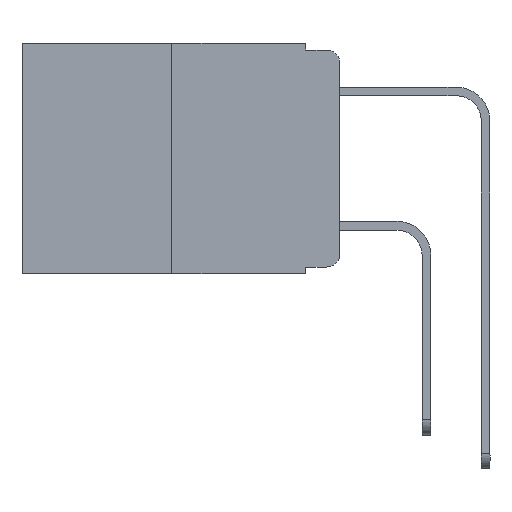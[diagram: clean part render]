
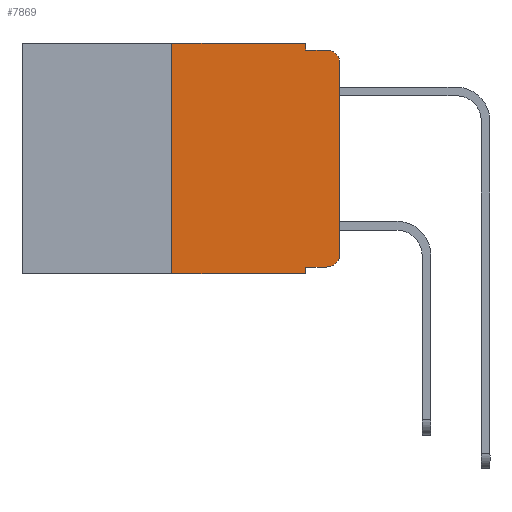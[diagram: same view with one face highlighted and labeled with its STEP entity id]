
A CAD part, left-side view. The second image highlights one B-rep face of the part: STEP entity #7869.
In plain terms, the highlighted planar face has unit normal (-1, 0, 0).
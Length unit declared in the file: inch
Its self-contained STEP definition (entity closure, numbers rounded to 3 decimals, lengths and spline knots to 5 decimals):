
#255 = VERTEX_POINT ( 'NONE', #11328 ) ;
#320 = CARTESIAN_POINT ( 'NONE',  ( 0., 0., -0.03 ) ) ;
#586 = LINE ( 'NONE', #3734, #12465 ) ;
#1014 = CARTESIAN_POINT ( 'NONE',  ( 0., 0.473, 0. ) ) ;
#1175 = VERTEX_POINT ( 'NONE', #11991 ) ;
#1264 = DIRECTION ( 'NONE',  ( 0., 0., -1. ) ) ;
#1426 = CARTESIAN_POINT ( 'NONE',  ( 0., 0.051, 0. ) ) ;
#1938 = VERTEX_POINT ( 'NONE', #16178 ) ;
#1976 = VERTEX_POINT ( 'NONE', #9786 ) ;
#2070 = ORIENTED_EDGE ( 'NONE', *, *, #16264, .F. ) ;
#2520 = VERTEX_POINT ( 'NONE', #320 ) ;
#2596 = CARTESIAN_POINT ( 'NONE',  ( 0., 0.473, 0. ) ) ;
#2667 = CARTESIAN_POINT ( 'NONE',  ( 0., 0.051, -0.01 ) ) ;
#2945 = DIRECTION ( 'NONE',  ( 0., -1., 0. ) ) ;
#3624 = VERTEX_POINT ( 'NONE', #10692 ) ;
#3734 = CARTESIAN_POINT ( 'NONE',  ( 0., 0.473, -0.343 ) ) ;
#3740 = DIRECTION ( 'NONE',  ( 0., 0., 1. ) ) ;
#4158 = VERTEX_POINT ( 'NONE', #15428 ) ;
#4434 = EDGE_CURVE ( 'NONE', #2520, #18762, #13626, .T. ) ;
#4568 = DIRECTION ( 'NONE',  ( 0., 0., -1. ) ) ;
#5041 = AXIS2_PLACEMENT_3D ( 'NONE', #15150, #12114, #19745 ) ;
#5365 = LINE ( 'NONE', #19301, #5650 ) ;
#5607 = DIRECTION ( 'NONE',  ( 0., -1., 0. ) ) ;
#5650 = VECTOR ( 'NONE', #7187, 39.37008 ) ;
#6432 = CARTESIAN_POINT ( 'NONE',  ( 0., 0.051, 0. ) ) ;
#6876 = EDGE_CURVE ( 'NONE', #10202, #1938, #14344, .T. ) ;
#7014 = EDGE_CURVE ( 'NONE', #1938, #18762, #8453, .T. ) ;
#7187 = DIRECTION ( 'NONE',  ( 0., 0., 1. ) ) ;
#7229 = ORIENTED_EDGE ( 'NONE', *, *, #7014, .F. ) ;
#7869 = ADVANCED_FACE ( 'NONE', ( #17148 ), #15623, .F. ) ;
#8090 = ORIENTED_EDGE ( 'NONE', *, *, #10468, .T. ) ;
#8453 = LINE ( 'NONE', #2667, #16938 ) ;
#9016 = VECTOR ( 'NONE', #3740, 39.37008 ) ;
#9132 = LINE ( 'NONE', #13785, #12609 ) ;
#9181 = DIRECTION ( 'NONE',  ( 0., -1., 0. ) ) ;
#9277 = ORIENTED_EDGE ( 'NONE', *, *, #6876, .F. ) ;
#9786 = CARTESIAN_POINT ( 'NONE',  ( 0., 0.25, 0. ) ) ;
#10202 = VERTEX_POINT ( 'NONE', #1426 ) ;
#10287 = CARTESIAN_POINT ( 'NONE',  ( 0., 0.02, -0.01 ) ) ;
#10468 = EDGE_CURVE ( 'NONE', #255, #4158, #586, .T. ) ;
#10527 = EDGE_CURVE ( 'NONE', #18423, #2520, #5365, .T. ) ;
#10692 = CARTESIAN_POINT ( 'NONE',  ( 0., 0.051, -0.333 ) ) ;
#10819 = CARTESIAN_POINT ( 'NONE',  ( 0., 0., -0.313 ) ) ;
#11205 = CIRCLE ( 'NONE', #5041, 0.02 ) ;
#11256 = ORIENTED_EDGE ( 'NONE', *, *, #19028, .F. ) ;
#11328 = CARTESIAN_POINT ( 'NONE',  ( 0., 0.25, -0.343 ) ) ;
#11362 = DIRECTION ( 'NONE',  ( -1., 0., 0. ) ) ;
#11364 = CARTESIAN_POINT ( 'NONE',  ( 0., 0.25, 0. ) ) ;
#11454 = CARTESIAN_POINT ( 'NONE',  ( 0., 0.02, -0.03 ) ) ;
#11749 = EDGE_CURVE ( 'NONE', #1175, #18423, #11205, .T. ) ;
#11991 = CARTESIAN_POINT ( 'NONE',  ( 0., 0.02, -0.333 ) ) ;
#12114 = DIRECTION ( 'NONE',  ( -1., 0., 0. ) ) ;
#12314 = ORIENTED_EDGE ( 'NONE', *, *, #17540, .F. ) ;
#12465 = VECTOR ( 'NONE', #12985, 39.37008 ) ;
#12473 = ORIENTED_EDGE ( 'NONE', *, *, #10527, .T. ) ;
#12609 = VECTOR ( 'NONE', #4568, 39.37008 ) ;
#12985 = DIRECTION ( 'NONE',  ( 0., -1., 0. ) ) ;
#13444 = LINE ( 'NONE', #19660, #14844 ) ;
#13626 = CIRCLE ( 'NONE', #13940, 0.02 ) ;
#13785 = CARTESIAN_POINT ( 'NONE',  ( 0., 0.051, 0. ) ) ;
#13940 = AXIS2_PLACEMENT_3D ( 'NONE', #11454, #11362, #16026 ) ;
#14017 = VECTOR ( 'NONE', #18837, 39.37008 ) ;
#14344 = LINE ( 'NONE', #6432, #14017 ) ;
#14844 = VECTOR ( 'NONE', #9181, 39.37008 ) ;
#15150 = CARTESIAN_POINT ( 'NONE',  ( 0., 0.02, -0.313 ) ) ;
#15269 = EDGE_CURVE ( 'NONE', #3624, #1175, #13444, .T. ) ;
#15335 = AXIS2_PLACEMENT_3D ( 'NONE', #2596, #18141, #1264 ) ;
#15428 = CARTESIAN_POINT ( 'NONE',  ( 0., 0.051, -0.343 ) ) ;
#15623 = PLANE ( 'NONE',  #15335 ) ;
#16026 = DIRECTION ( 'NONE',  ( 0., 0., -1. ) ) ;
#16100 = VECTOR ( 'NONE', #2945, 39.37008 ) ;
#16178 = CARTESIAN_POINT ( 'NONE',  ( 0., 0.051, -0.01 ) ) ;
#16264 = EDGE_CURVE ( 'NONE', #3624, #4158, #9132, .T. ) ;
#16657 = LINE ( 'NONE', #1014, #16100 ) ;
#16938 = VECTOR ( 'NONE', #5607, 39.37008 ) ;
#17087 = ORIENTED_EDGE ( 'NONE', *, *, #11749, .T. ) ;
#17148 = FACE_OUTER_BOUND ( 'NONE', #19025, .T. ) ;
#17540 = EDGE_CURVE ( 'NONE', #1976, #10202, #16657, .T. ) ;
#17725 = ORIENTED_EDGE ( 'NONE', *, *, #4434, .T. ) ;
#18141 = DIRECTION ( 'NONE',  ( 1., 0., 0. ) ) ;
#18423 = VERTEX_POINT ( 'NONE', #10819 ) ;
#18762 = VERTEX_POINT ( 'NONE', #10287 ) ;
#18837 = DIRECTION ( 'NONE',  ( 0., 0., -1. ) ) ;
#19025 = EDGE_LOOP ( 'NONE', ( #12473, #17725, #7229, #9277, #12314, #11256, #8090, #2070, #19159, #17087 ) ) ;
#19028 = EDGE_CURVE ( 'NONE', #255, #1976, #19103, .T. ) ;
#19103 = LINE ( 'NONE', #11364, #9016 ) ;
#19159 = ORIENTED_EDGE ( 'NONE', *, *, #15269, .T. ) ;
#19301 = CARTESIAN_POINT ( 'NONE',  ( 0., 0., 0. ) ) ;
#19660 = CARTESIAN_POINT ( 'NONE',  ( 0., 0.051, -0.333 ) ) ;
#19745 = DIRECTION ( 'NONE',  ( 0., 0., -1. ) ) ;
